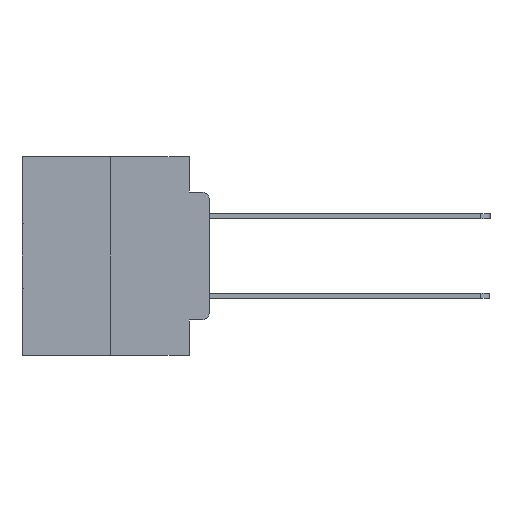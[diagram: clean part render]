
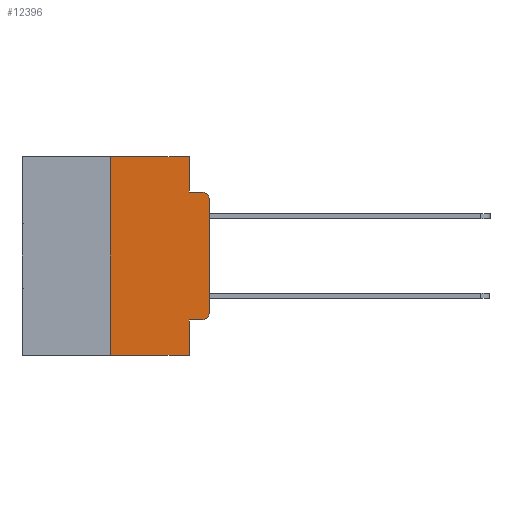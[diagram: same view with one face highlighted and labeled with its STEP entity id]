
A CAD part, left-side view. The second image highlights one B-rep face of the part: STEP entity #12396.
In plain terms, the highlighted planar face has unit normal (-1, 0, 0).
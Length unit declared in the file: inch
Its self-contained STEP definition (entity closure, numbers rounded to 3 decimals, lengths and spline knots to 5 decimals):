
#194 = DIRECTION ( 'NONE',  ( 1., 0., 0. ) ) ;
#701 = CARTESIAN_POINT ( 'NONE',  ( 0., 0.051, 0. ) ) ;
#1420 = EDGE_CURVE ( 'NONE', #9401, #16187, #10704, .T. ) ;
#1790 = CARTESIAN_POINT ( 'NONE',  ( 0., 0.02, -0.0885 ) ) ;
#2202 = ORIENTED_EDGE ( 'NONE', *, *, #28862, .T. ) ;
#3059 = EDGE_CURVE ( 'NONE', #16187, #26873, #30022, .T. ) ;
#3066 = FACE_OUTER_BOUND ( 'NONE', #27157, .T. ) ;
#3384 = CARTESIAN_POINT ( 'NONE',  ( 0., 0.051, -0.4115 ) ) ;
#3792 = AXIS2_PLACEMENT_3D ( 'NONE', #8298, #25070, #10741 ) ;
#3973 = EDGE_CURVE ( 'NONE', #9405, #12044, #15919, .T. ) ;
#4083 = ORIENTED_EDGE ( 'NONE', *, *, #1420, .T. ) ;
#4147 = ORIENTED_EDGE ( 'NONE', *, *, #3973, .T. ) ;
#4222 = VECTOR ( 'NONE', #10212, 39.37008 ) ;
#4267 = VECTOR ( 'NONE', #17430, 39.37008 ) ;
#5808 = DIRECTION ( 'NONE',  ( -1., 0., 0. ) ) ;
#6226 = AXIS2_PLACEMENT_3D ( 'NONE', #14795, #194, #17163 ) ;
#7386 = CARTESIAN_POINT ( 'NONE',  ( 0., 0.473, -0.5 ) ) ;
#7526 = PLANE ( 'NONE',  #6226 ) ;
#8016 = LINE ( 'NONE', #23182, #19982 ) ;
#8298 = CARTESIAN_POINT ( 'NONE',  ( 0., 0.02, -0.1085 ) ) ;
#8550 = VECTOR ( 'NONE', #20233, 39.37008 ) ;
#9084 = LINE ( 'NONE', #21399, #14710 ) ;
#9270 = VECTOR ( 'NONE', #24916, 39.37008 ) ;
#9401 = VERTEX_POINT ( 'NONE', #28427 ) ;
#9405 = VERTEX_POINT ( 'NONE', #16599 ) ;
#9559 = VECTOR ( 'NONE', #24174, 39.37008 ) ;
#9630 = EDGE_CURVE ( 'NONE', #16675, #26873, #11482, .T. ) ;
#9680 = VERTEX_POINT ( 'NONE', #24785 ) ;
#10045 = LINE ( 'NONE', #701, #9270 ) ;
#10212 = DIRECTION ( 'NONE',  ( 0., 0., 1. ) ) ;
#10704 = LINE ( 'NONE', #13746, #4222 ) ;
#10741 = DIRECTION ( 'NONE',  ( 0., 0., -1. ) ) ;
#11234 = EDGE_CURVE ( 'NONE', #18745, #16675, #10045, .T. ) ;
#11482 = LINE ( 'NONE', #24572, #4267 ) ;
#11716 = CARTESIAN_POINT ( 'NONE',  ( 0., 0.25, 0. ) ) ;
#11899 = DIRECTION ( 'NONE',  ( 0., 0., -1. ) ) ;
#12044 = VERTEX_POINT ( 'NONE', #18254 ) ;
#12396 = ADVANCED_FACE ( 'NONE', ( #3066 ), #7526, .F. ) ;
#12555 = VECTOR ( 'NONE', #28447, 39.37008 ) ;
#12716 = CARTESIAN_POINT ( 'NONE',  ( 0., 0.051, 0. ) ) ;
#12853 = EDGE_CURVE ( 'NONE', #9405, #13936, #22265, .T. ) ;
#13746 = CARTESIAN_POINT ( 'NONE',  ( 0., 0., 0. ) ) ;
#13936 = VERTEX_POINT ( 'NONE', #29839 ) ;
#14076 = EDGE_CURVE ( 'NONE', #13936, #18745, #8016, .T. ) ;
#14710 = VECTOR ( 'NONE', #11899, 39.37008 ) ;
#14725 = ORIENTED_EDGE ( 'NONE', *, *, #12853, .F. ) ;
#14795 = CARTESIAN_POINT ( 'NONE',  ( 0., 0.473, 0. ) ) ;
#15919 = LINE ( 'NONE', #7386, #9559 ) ;
#16134 = CIRCLE ( 'NONE', #26264, 0.02 ) ;
#16187 = VERTEX_POINT ( 'NONE', #26594 ) ;
#16599 = CARTESIAN_POINT ( 'NONE',  ( 0., 0.25, -0.5 ) ) ;
#16675 = VERTEX_POINT ( 'NONE', #19219 ) ;
#17163 = DIRECTION ( 'NONE',  ( 0., 0., -1. ) ) ;
#17430 = DIRECTION ( 'NONE',  ( 0., -1., 0. ) ) ;
#17641 = ORIENTED_EDGE ( 'NONE', *, *, #3059, .T. ) ;
#18254 = CARTESIAN_POINT ( 'NONE',  ( 0., 0.051, -0.5 ) ) ;
#18745 = VERTEX_POINT ( 'NONE', #12716 ) ;
#19219 = CARTESIAN_POINT ( 'NONE',  ( 0., 0.051, -0.0885 ) ) ;
#19982 = VECTOR ( 'NONE', #27985, 39.37008 ) ;
#20154 = CARTESIAN_POINT ( 'NONE',  ( 0., 0.02, -0.3915 ) ) ;
#20233 = DIRECTION ( 'NONE',  ( 0., -1., 0. ) ) ;
#20703 = ORIENTED_EDGE ( 'NONE', *, *, #27280, .T. ) ;
#21399 = CARTESIAN_POINT ( 'NONE',  ( 0., 0.051, 0. ) ) ;
#22265 = LINE ( 'NONE', #11716, #12555 ) ;
#22598 = DIRECTION ( 'NONE',  ( 0., 0., -1. ) ) ;
#23182 = CARTESIAN_POINT ( 'NONE',  ( 0., 0.473, 0. ) ) ;
#24027 = ORIENTED_EDGE ( 'NONE', *, *, #9630, .F. ) ;
#24074 = EDGE_CURVE ( 'NONE', #24399, #12044, #9084, .T. ) ;
#24092 = ORIENTED_EDGE ( 'NONE', *, *, #24074, .F. ) ;
#24174 = DIRECTION ( 'NONE',  ( 0., -1., 0. ) ) ;
#24399 = VERTEX_POINT ( 'NONE', #24982 ) ;
#24572 = CARTESIAN_POINT ( 'NONE',  ( 0., 0.051, -0.0885 ) ) ;
#24785 = CARTESIAN_POINT ( 'NONE',  ( 0., 0.02, -0.4115 ) ) ;
#24916 = DIRECTION ( 'NONE',  ( 0., 0., -1. ) ) ;
#24982 = CARTESIAN_POINT ( 'NONE',  ( 0., 0.051, -0.4115 ) ) ;
#25070 = DIRECTION ( 'NONE',  ( -1., 0., 0. ) ) ;
#25935 = ORIENTED_EDGE ( 'NONE', *, *, #14076, .F. ) ;
#26136 = LINE ( 'NONE', #3384, #8550 ) ;
#26264 = AXIS2_PLACEMENT_3D ( 'NONE', #20154, #5808, #22598 ) ;
#26594 = CARTESIAN_POINT ( 'NONE',  ( 0., 0., -0.1085 ) ) ;
#26873 = VERTEX_POINT ( 'NONE', #1790 ) ;
#27157 = EDGE_LOOP ( 'NONE', ( #4083, #17641, #24027, #30744, #25935, #14725, #4147, #24092, #20703, #2202 ) ) ;
#27280 = EDGE_CURVE ( 'NONE', #24399, #9680, #26136, .T. ) ;
#27985 = DIRECTION ( 'NONE',  ( 0., -1., 0. ) ) ;
#28427 = CARTESIAN_POINT ( 'NONE',  ( 0., 0., -0.3915 ) ) ;
#28447 = DIRECTION ( 'NONE',  ( 0., 0., 1. ) ) ;
#28862 = EDGE_CURVE ( 'NONE', #9680, #9401, #16134, .T. ) ;
#29839 = CARTESIAN_POINT ( 'NONE',  ( 0., 0.25, 0. ) ) ;
#30022 = CIRCLE ( 'NONE', #3792, 0.02 ) ;
#30744 = ORIENTED_EDGE ( 'NONE', *, *, #11234, .F. ) ;
